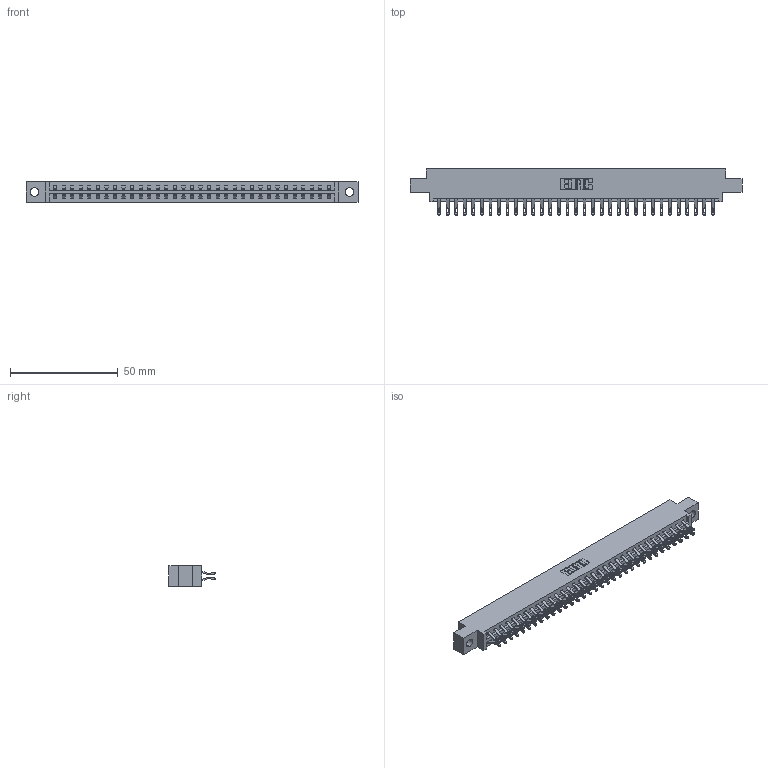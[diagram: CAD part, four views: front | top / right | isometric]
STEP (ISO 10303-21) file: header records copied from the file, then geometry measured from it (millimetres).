
FILE_DESCRIPTION (( 'STEP AP203' ), '1' );
FILE_NAME ('387-066-555-804.STEP', '2018-09-21T11:23:11', ( '' ), ( '' ), 'SwSTEP 2.0', 'SolidWorks 2016', '' );
FILE_SCHEMA (( 'CONFIG_CONTROL_DESIGN' ));
Length unit declared in the file: inch
Products named in the file (3): 337 Part_0.170 Offset - 0.156 Dia-TH; 345-292-001_555 Tail; 387-066-555-804
Assembly tree (67 placements, depth 2):
  387-066-555-804
    337 Part_0.170 Offset - 0.156 Dia-TH
    345-292-001_555 Tail  x66
Bounding box: 153.77 x 21.47 x 9.4 mm (x, y, z)
Volume: 16071.9 mm3; surface area: 18708.6 mm2
Topology: 67 solids, 67 shells, 4078 faces, 12797 edges, 8530 vertices
Faces by surface type: plane 2450, cylinder 1628
Entity records: 27211 total; most frequent: CARTESIAN_POINT 4628, ORIENTED_EDGE 4534, DIRECTION 3923, EDGE_CURVE 2267, LINE 2119, VECTOR 2119, VERTEX_POINT 1510, AXIS2_PLACEMENT_3D 902
